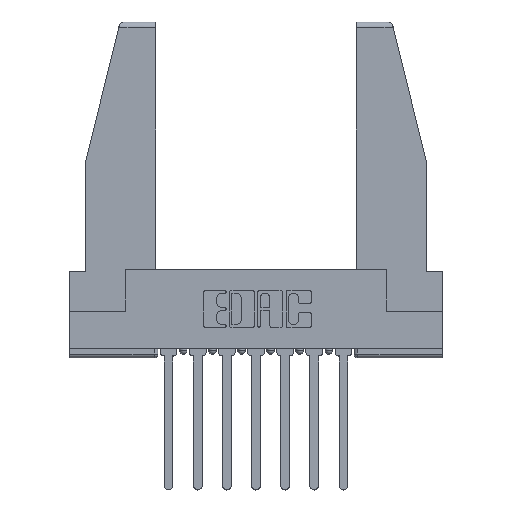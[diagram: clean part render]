
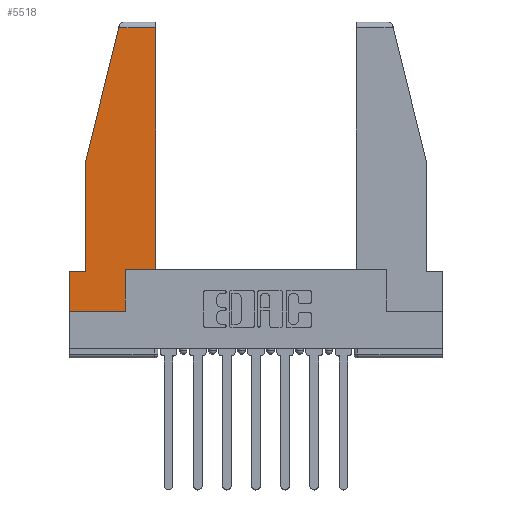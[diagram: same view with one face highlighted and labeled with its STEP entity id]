
A CAD part, top view. The second image highlights one B-rep face of the part: STEP entity #5518.
In plain terms, the highlighted planar face has unit normal (0, 0, 1).
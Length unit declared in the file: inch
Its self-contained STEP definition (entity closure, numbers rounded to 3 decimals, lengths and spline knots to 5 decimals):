
#119 = VERTEX_POINT ( 'NONE', #2973 ) ;
#200 = VERTEX_POINT ( 'NONE', #12503 ) ;
#375 = ORIENTED_EDGE ( 'NONE', *, *, #8611, .T. ) ;
#409 = EDGE_CURVE ( 'NONE', #200, #6071, #2701, .T. ) ;
#496 = LINE ( 'NONE', #5061, #11788 ) ;
#550 = EDGE_CURVE ( 'NONE', #119, #4381, #496, .T. ) ;
#555 = CARTESIAN_POINT ( 'NONE',  ( 0.086, 0.21, 0. ) ) ;
#634 = LINE ( 'NONE', #11851, #6259 ) ;
#751 = CARTESIAN_POINT ( 'NONE',  ( 0.461, 1.52, 0. ) ) ;
#1248 = ORIENTED_EDGE ( 'NONE', *, *, #550, .T. ) ;
#1305 = ORIENTED_EDGE ( 'NONE', *, *, #10384, .T. ) ;
#1336 = DIRECTION ( 'NONE',  ( 1., 0., 0. ) ) ;
#1353 = LINE ( 'NONE', #7319, #11701 ) ;
#1669 = AXIS2_PLACEMENT_3D ( 'NONE', #4820, #11923, #12922 ) ;
#1989 = DIRECTION ( 'NONE',  ( 0., 1., 0. ) ) ;
#2235 = LINE ( 'NONE', #4713, #12108 ) ;
#2669 = EDGE_CURVE ( 'NONE', #4381, #6021, #4816, .T. ) ;
#2701 = LINE ( 'NONE', #3576, #12427 ) ;
#2934 = DIRECTION ( 'NONE',  ( 0., -1., 0. ) ) ;
#2973 = CARTESIAN_POINT ( 'NONE',  ( 0.297, 0., 0. ) ) ;
#3576 = CARTESIAN_POINT ( 'NONE',  ( 0., 0.21, 0. ) ) ;
#3665 = ORIENTED_EDGE ( 'NONE', *, *, #409, .T. ) ;
#3794 = ORIENTED_EDGE ( 'NONE', *, *, #5291, .T. ) ;
#3817 = ORIENTED_EDGE ( 'NONE', *, *, #6248, .T. ) ;
#3837 = PLANE ( 'NONE',  #1669 ) ;
#4324 = CARTESIAN_POINT ( 'NONE',  ( 0.297, 0.223, 0. ) ) ;
#4381 = VERTEX_POINT ( 'NONE', #9614 ) ;
#4398 = VERTEX_POINT ( 'NONE', #751 ) ;
#4475 = CARTESIAN_POINT ( 'NONE',  ( 0.271, 1.55, 0. ) ) ;
#4713 = CARTESIAN_POINT ( 'NONE',  ( 0., 1.52, 0. ) ) ;
#4816 = LINE ( 'NONE', #4324, #9815 ) ;
#4820 = CARTESIAN_POINT ( 'NONE',  ( 0., 0., 0. ) ) ;
#4891 = DIRECTION ( 'NONE',  ( 0., 1., 0. ) ) ;
#5061 = CARTESIAN_POINT ( 'NONE',  ( 0.297, 0., 0. ) ) ;
#5291 = EDGE_CURVE ( 'NONE', #6021, #4398, #11455, .T. ) ;
#5307 = ORIENTED_EDGE ( 'NONE', *, *, #2669, .T. ) ;
#5472 = DIRECTION ( 'NONE',  ( -1., 0., 0. ) ) ;
#5518 = ADVANCED_FACE ( 'NONE', ( #9066 ), #3837, .T. ) ;
#5535 = EDGE_CURVE ( 'NONE', #8457, #10845, #634, .T. ) ;
#5834 = VERTEX_POINT ( 'NONE', #9653 ) ;
#6021 = VERTEX_POINT ( 'NONE', #7504 ) ;
#6071 = VERTEX_POINT ( 'NONE', #9651 ) ;
#6248 = EDGE_CURVE ( 'NONE', #10845, #200, #7932, .T. ) ;
#6259 = VECTOR ( 'NONE', #2934, 39.37008 ) ;
#6335 = DIRECTION ( 'NONE',  ( 1., 0., 0. ) ) ;
#7319 = CARTESIAN_POINT ( 'NONE',  ( 0., 0., 0. ) ) ;
#7504 = CARTESIAN_POINT ( 'NONE',  ( 0.461, 0.223, 0. ) ) ;
#7932 = LINE ( 'NONE', #9422, #10798 ) ;
#8457 = VERTEX_POINT ( 'NONE', #12238 ) ;
#8495 = DIRECTION ( 'NONE',  ( 0., -1., 0. ) ) ;
#8611 = EDGE_CURVE ( 'NONE', #6071, #119, #1353, .T. ) ;
#9066 = FACE_OUTER_BOUND ( 'NONE', #9071, .T. ) ;
#9071 = EDGE_LOOP ( 'NONE', ( #3794, #1305, #9769, #12838, #3817, #3665, #375, #1248, #5307 ) ) ;
#9239 = VECTOR ( 'NONE', #4891, 39.37008 ) ;
#9411 = DIRECTION ( 'NONE',  ( -0.239, -0.971, 0. ) ) ;
#9422 = CARTESIAN_POINT ( 'NONE',  ( 0., 0.21, 0. ) ) ;
#9614 = CARTESIAN_POINT ( 'NONE',  ( 0.297, 0.223, 0. ) ) ;
#9622 = EDGE_CURVE ( 'NONE', #5834, #8457, #10414, .T. ) ;
#9651 = CARTESIAN_POINT ( 'NONE',  ( 0., 0., 0. ) ) ;
#9653 = CARTESIAN_POINT ( 'NONE',  ( 0.2636, 1.52, 0. ) ) ;
#9769 = ORIENTED_EDGE ( 'NONE', *, *, #9622, .T. ) ;
#9815 = VECTOR ( 'NONE', #6335, 39.37008 ) ;
#10243 = VECTOR ( 'NONE', #9411, 39.37008 ) ;
#10384 = EDGE_CURVE ( 'NONE', #4398, #5834, #2235, .T. ) ;
#10414 = LINE ( 'NONE', #4475, #10243 ) ;
#10607 = CARTESIAN_POINT ( 'NONE',  ( 0.461, 0.223, 0. ) ) ;
#10798 = VECTOR ( 'NONE', #5472, 39.37008 ) ;
#10845 = VERTEX_POINT ( 'NONE', #555 ) ;
#11455 = LINE ( 'NONE', #10607, #9239 ) ;
#11701 = VECTOR ( 'NONE', #1336, 39.37008 ) ;
#11781 = DIRECTION ( 'NONE',  ( -1., 0., 0. ) ) ;
#11788 = VECTOR ( 'NONE', #1989, 39.37008 ) ;
#11851 = CARTESIAN_POINT ( 'NONE',  ( 0.086, 0.8, 0. ) ) ;
#11923 = DIRECTION ( 'NONE',  ( 0., 0., 1. ) ) ;
#12108 = VECTOR ( 'NONE', #11781, 39.37008 ) ;
#12238 = CARTESIAN_POINT ( 'NONE',  ( 0.086, 0.8, 0. ) ) ;
#12427 = VECTOR ( 'NONE', #8495, 39.37008 ) ;
#12503 = CARTESIAN_POINT ( 'NONE',  ( 0., 0.21, 0. ) ) ;
#12838 = ORIENTED_EDGE ( 'NONE', *, *, #5535, .T. ) ;
#12922 = DIRECTION ( 'NONE',  ( 1., 0., 0. ) ) ;
